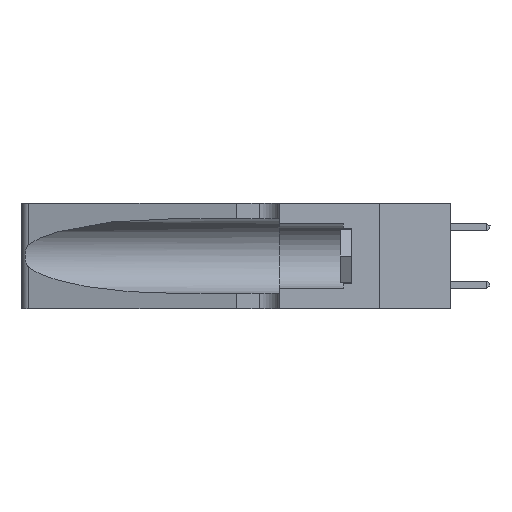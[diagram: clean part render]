
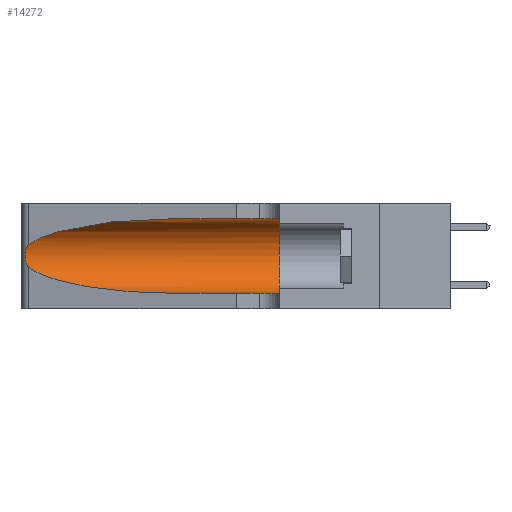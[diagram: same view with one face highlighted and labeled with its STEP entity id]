
A CAD part, left-side view. The second image highlights one B-rep face of the part: STEP entity #14272.
In plain terms, the highlighted cylindrical face has radius 3.308 mm (diameter 6.617 mm), a partial arc.
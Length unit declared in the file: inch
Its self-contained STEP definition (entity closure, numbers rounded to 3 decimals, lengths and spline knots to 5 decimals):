
#361 = EDGE_CURVE ( 'NONE', #6732, #2976, #11117, .T. ) ;
#378 = VERTEX_POINT ( 'NONE', #16548 ) ;
#688 = CARTESIAN_POINT ( 'NONE',  ( 0.1305, 0.35, 0.05475 ) ) ;
#714 = EDGE_LOOP ( 'NONE', ( #25699, #2601, #28182, #10990, #21802, #28314 ) ) ;
#754 = DIRECTION ( 'NONE',  ( 0., -1., 0. ) ) ;
#839 = CARTESIAN_POINT ( 'NONE',  ( 0.25555, 1.22994, 0.2215 ) ) ;
#952 = EDGE_CURVE ( 'NONE', #17202, #25769, #5914, .T. ) ;
#1041 = CARTESIAN_POINT ( 'NONE',  ( 0.25856, 1.23593, 0.16098 ) ) ;
#2008 = CARTESIAN_POINT ( 'NONE',  ( 0.2373, 1.15595, 0.28018 ) ) ;
#2601 = ORIENTED_EDGE ( 'NONE', *, *, #3898, .T. ) ;
#2768 = CARTESIAN_POINT ( 'NONE',  ( 0.25487, 1.22718, 0.14631 ) ) ;
#2905 = AXIS2_PLACEMENT_3D ( 'NONE', #5854, #10373, #21278 ) ;
#2976 = VERTEX_POINT ( 'NONE', #17393 ) ;
#3352 = CARTESIAN_POINT ( 'NONE',  ( 0.25639, 1.23186, 0.15144 ) ) ;
#3898 = EDGE_CURVE ( 'NONE', #2976, #17202, #24276, .T. ) ;
#5458 = CYLINDRICAL_SURFACE ( 'NONE', #2905, 0.13025 ) ;
#5632 = CARTESIAN_POINT ( 'NONE',  ( 0.25487, 1.22718, 0.14631 ) ) ;
#5854 = CARTESIAN_POINT ( 'NONE',  ( 0.1305, 1.61858, 0.185 ) ) ;
#5914 =( BOUNDED_CURVE ( )  B_SPLINE_CURVE ( 3, ( #16537, #22308, #23105, #25753 ),
 .UNSPECIFIED., .F., .F. ) 
 B_SPLINE_CURVE_WITH_KNOTS ( ( 4, 4 ),
 ( 3.44316, 4.71239 ),
 .UNSPECIFIED. ) 
 CURVE ( )  GEOMETRIC_REPRESENTATION_ITEM ( )  RATIONAL_B_SPLINE_CURVE ( ( 1., 0.87, 0.87, 1. ) ) 
 REPRESENTATION_ITEM ( '' )  );
#5953 = VERTEX_POINT ( 'NONE', #688 ) ;
#6732 = VERTEX_POINT ( 'NONE', #7826 ) ;
#6826 = DIRECTION ( 'NONE',  ( 0., 1., 0. ) ) ;
#7507 = CIRCLE ( 'NONE', #22488, 0.13025 ) ;
#7808 = CARTESIAN_POINT ( 'NONE',  ( 0.25639, 1.23184, 0.21858 ) ) ;
#7826 = CARTESIAN_POINT ( 'NONE',  ( 0.1305, 0.72297, 0.31525 ) ) ;
#9759 = EDGE_CURVE ( 'NONE', #378, #5953, #7507, .T. ) ;
#10053 = CARTESIAN_POINT ( 'NONE',  ( 0.25854, 1.2359, 0.20912 ) ) ;
#10373 = DIRECTION ( 'NONE',  ( 0., -1., 0. ) ) ;
#10990 = ORIENTED_EDGE ( 'NONE', *, *, #23700, .T. ) ;
#11117 =( BOUNDED_CURVE ( )  B_SPLINE_CURVE ( 3, ( #23517, #23225, #2008, #17294 ),
 .UNSPECIFIED., .F., .T. ) 
 B_SPLINE_CURVE_WITH_KNOTS ( ( 4, 4 ),
 ( 1.5708, 2.84003 ),
 .UNSPECIFIED. ) 
 CURVE ( )  GEOMETRIC_REPRESENTATION_ITEM ( )  RATIONAL_B_SPLINE_CURVE ( ( 1., 0.87, 0.87, 1. ) ) 
 REPRESENTATION_ITEM ( '' )  );
#12273 = CARTESIAN_POINT ( 'NONE',  ( 0.26075, 1.23896, 0.19203 ) ) ;
#14210 = CARTESIAN_POINT ( 'NONE',  ( 0.1305, 1.61858, 0.31525 ) ) ;
#14272 = ADVANCED_FACE ( 'NONE', ( #17913 ), #5458, .F. ) ;
#14488 = CARTESIAN_POINT ( 'NONE',  ( 0.26017, 1.23833, 0.17102 ) ) ;
#14582 = DIRECTION ( 'NONE',  ( 0., -1., 0. ) ) ;
#16537 = CARTESIAN_POINT ( 'NONE',  ( 0.25487, 1.22718, 0.14631 ) ) ;
#16548 = CARTESIAN_POINT ( 'NONE',  ( 0.1305, 0.35, 0.31525 ) ) ;
#16597 = CARTESIAN_POINT ( 'NONE',  ( 0.25487, 1.22718, 0.22369 ) ) ;
#16694 = CARTESIAN_POINT ( 'NONE',  ( 0.25789, 1.23486, 0.15765 ) ) ;
#17202 = VERTEX_POINT ( 'NONE', #2768 ) ;
#17294 = CARTESIAN_POINT ( 'NONE',  ( 0.25487, 1.22718, 0.22369 ) ) ;
#17393 = CARTESIAN_POINT ( 'NONE',  ( 0.25487, 1.22718, 0.22369 ) ) ;
#17913 = FACE_OUTER_BOUND ( 'NONE', #714, .T. ) ;
#18506 = LINE ( 'NONE', #18959, #22251 ) ;
#18878 = CARTESIAN_POINT ( 'NONE',  ( 0.25555, 1.22993, 0.14849 ) ) ;
#18959 = CARTESIAN_POINT ( 'NONE',  ( 0.1305, 1.61858, 0.05475 ) ) ;
#20048 = CARTESIAN_POINT ( 'NONE',  ( 0.1305, 0.35, 0.185 ) ) ;
#20760 = EDGE_CURVE ( 'NONE', #6732, #378, #28620, .T. ) ;
#21278 = DIRECTION ( 'NONE',  ( 0., 0., -1. ) ) ;
#21802 = ORIENTED_EDGE ( 'NONE', *, *, #9759, .F. ) ;
#22232 = DIRECTION ( 'NONE',  ( 0., 0., 1. ) ) ;
#22251 = VECTOR ( 'NONE', #14582, 39.37008 ) ;
#22308 = CARTESIAN_POINT ( 'NONE',  ( 0.2373, 1.15595, 0.08982 ) ) ;
#22488 = AXIS2_PLACEMENT_3D ( 'NONE', #20048, #6826, #22232 ) ;
#23105 = CARTESIAN_POINT ( 'NONE',  ( 0.18966, 0.96281, 0.05475 ) ) ;
#23162 = CARTESIAN_POINT ( 'NONE',  ( 0.25787, 1.23484, 0.2124 ) ) ;
#23225 = CARTESIAN_POINT ( 'NONE',  ( 0.18966, 0.96281, 0.31525 ) ) ;
#23517 = CARTESIAN_POINT ( 'NONE',  ( 0.1305, 0.72297, 0.31525 ) ) ;
#23549 = VECTOR ( 'NONE', #754, 39.37008 ) ;
#23700 = EDGE_CURVE ( 'NONE', #25769, #5953, #18506, .T. ) ;
#24276 = B_SPLINE_CURVE_WITH_KNOTS ( 'NONE', 3,
 ( #16597, #839, #7808, #23162, #10053, #25342, #12273, #27524, #14488, #1041, #16694, #3352, #18878, #5632 ),
 .UNSPECIFIED., .F., .F.,
 ( 4, 2, 2, 2, 2, 2, 4 ),
 ( 0., 0.00027, 0.00053, 0.00107, 0.0016, 0.00187, 0.00214 ),
 .UNSPECIFIED. ) ;
#25342 = CARTESIAN_POINT ( 'NONE',  ( 0.26018, 1.23835, 0.19895 ) ) ;
#25699 = ORIENTED_EDGE ( 'NONE', *, *, #361, .T. ) ;
#25753 = CARTESIAN_POINT ( 'NONE',  ( 0.1305, 0.72297, 0.05475 ) ) ;
#25769 = VERTEX_POINT ( 'NONE', #28270 ) ;
#27524 = CARTESIAN_POINT ( 'NONE',  ( 0.26075, 1.23896, 0.178 ) ) ;
#28182 = ORIENTED_EDGE ( 'NONE', *, *, #952, .T. ) ;
#28270 = CARTESIAN_POINT ( 'NONE',  ( 0.1305, 0.72297, 0.05475 ) ) ;
#28314 = ORIENTED_EDGE ( 'NONE', *, *, #20760, .F. ) ;
#28620 = LINE ( 'NONE', #14210, #23549 ) ;
